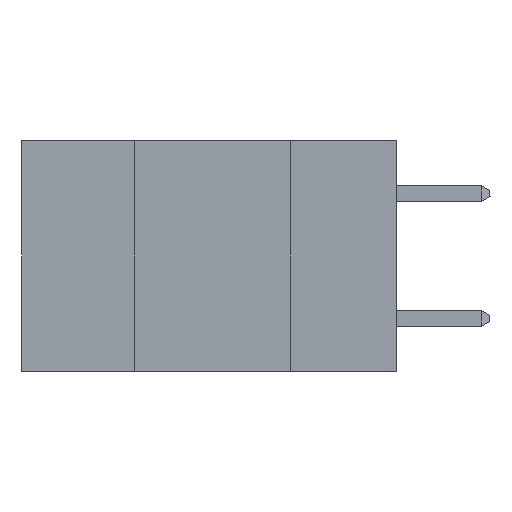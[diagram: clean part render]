
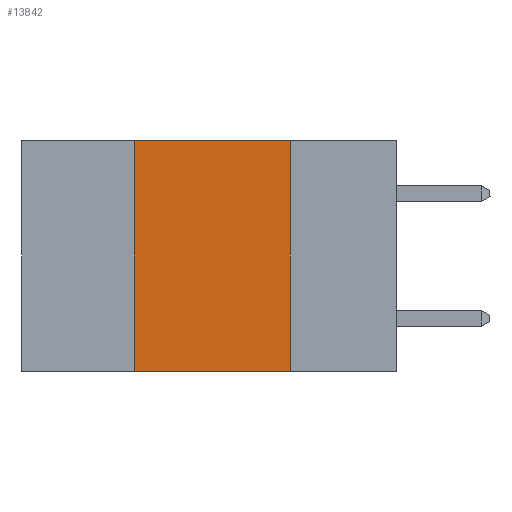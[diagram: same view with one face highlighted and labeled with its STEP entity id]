
A CAD part, left-side view. The second image highlights one B-rep face of the part: STEP entity #13842.
In plain terms, the highlighted planar face has unit normal (-1, 0, 0).
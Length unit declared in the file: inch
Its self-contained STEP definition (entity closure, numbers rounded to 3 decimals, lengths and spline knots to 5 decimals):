
#272 = LINE ( 'NONE', #12004, #12306 ) ;
#518 = CARTESIAN_POINT ( 'NONE',  ( 0., 0.6, -0.37 ) ) ;
#582 = DIRECTION ( 'NONE',  ( 0., -1., 0. ) ) ;
#961 = DIRECTION ( 'NONE',  ( 0., 0., -1. ) ) ;
#995 = VERTEX_POINT ( 'NONE', #1417 ) ;
#1417 = CARTESIAN_POINT ( 'NONE',  ( 0., 0.42, 0. ) ) ;
#2097 = EDGE_CURVE ( 'NONE', #7408, #995, #16335, .T. ) ;
#3456 = FACE_OUTER_BOUND ( 'NONE', #15494, .T. ) ;
#3549 = ORIENTED_EDGE ( 'NONE', *, *, #17759, .F. ) ;
#4127 = CARTESIAN_POINT ( 'NONE',  ( 0., 0.17, 0. ) ) ;
#5430 = VERTEX_POINT ( 'NONE', #18567 ) ;
#7408 = VERTEX_POINT ( 'NONE', #7760 ) ;
#7508 = VECTOR ( 'NONE', #11373, 39.37008 ) ;
#7760 = CARTESIAN_POINT ( 'NONE',  ( 0., 0.42, -0.37 ) ) ;
#8999 = AXIS2_PLACEMENT_3D ( 'NONE', #16026, #15961, #11214 ) ;
#9334 = EDGE_CURVE ( 'NONE', #5430, #19331, #18603, .T. ) ;
#9383 = PLANE ( 'NONE',  #8999 ) ;
#9394 = LINE ( 'NONE', #518, #11095 ) ;
#9410 = ORIENTED_EDGE ( 'NONE', *, *, #2097, .F. ) ;
#10749 = VECTOR ( 'NONE', #961, 39.37008 ) ;
#11095 = VECTOR ( 'NONE', #582, 39.37008 ) ;
#11214 = DIRECTION ( 'NONE',  ( 0., 0., -1. ) ) ;
#11373 = DIRECTION ( 'NONE',  ( 0., 0., 1. ) ) ;
#11505 = CARTESIAN_POINT ( 'NONE',  ( 0., 0.42, 0. ) ) ;
#11935 = DIRECTION ( 'NONE',  ( 0., -1., 0. ) ) ;
#12004 = CARTESIAN_POINT ( 'NONE',  ( 0., 0.6, 0. ) ) ;
#12306 = VECTOR ( 'NONE', #11935, 39.37008 ) ;
#13842 = ADVANCED_FACE ( 'NONE', ( #3456 ), #9383, .F. ) ;
#14120 = ORIENTED_EDGE ( 'NONE', *, *, #16304, .T. ) ;
#15494 = EDGE_LOOP ( 'NONE', ( #19178, #3549, #9410, #14120 ) ) ;
#15961 = DIRECTION ( 'NONE',  ( 1., 0., 0. ) ) ;
#16026 = CARTESIAN_POINT ( 'NONE',  ( 0., 0.6, 0. ) ) ;
#16304 = EDGE_CURVE ( 'NONE', #7408, #19331, #9394, .T. ) ;
#16335 = LINE ( 'NONE', #11505, #7508 ) ;
#17523 = CARTESIAN_POINT ( 'NONE',  ( 0., 0.17, -0.37 ) ) ;
#17759 = EDGE_CURVE ( 'NONE', #995, #5430, #272, .T. ) ;
#18567 = CARTESIAN_POINT ( 'NONE',  ( 0., 0.17, 0. ) ) ;
#18603 = LINE ( 'NONE', #4127, #10749 ) ;
#19178 = ORIENTED_EDGE ( 'NONE', *, *, #9334, .F. ) ;
#19331 = VERTEX_POINT ( 'NONE', #17523 ) ;
